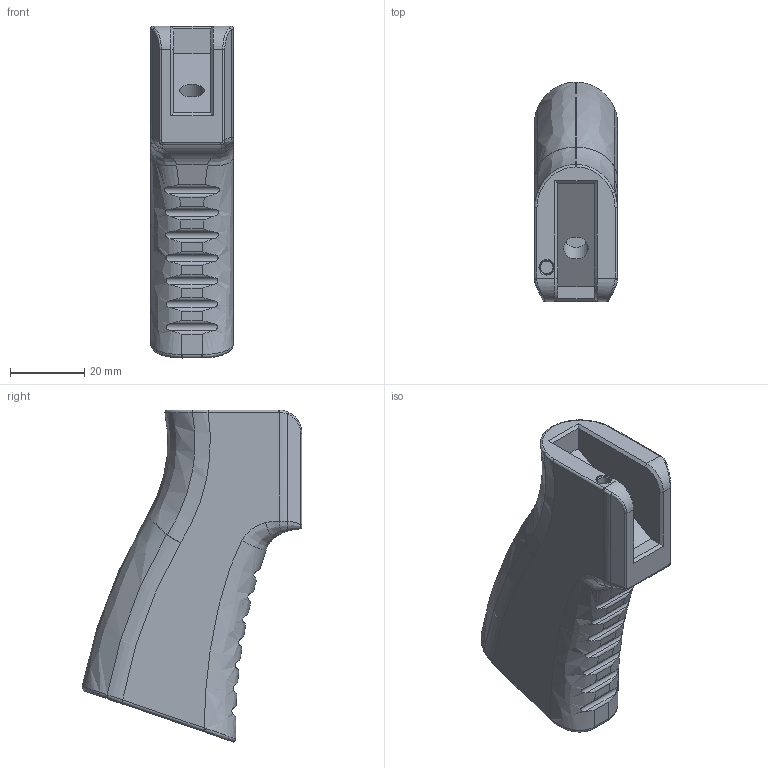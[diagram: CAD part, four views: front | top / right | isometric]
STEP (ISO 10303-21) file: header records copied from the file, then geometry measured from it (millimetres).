
FILE_DESCRIPTION(/* description */ (''),/* implementation_level */ '2;1');
FILE_NAME(/* name */ 'Vulpes Grip.step',/* time_stamp */ '2021-10-04T05:32:21-04:00',/* author */ (''),/* organization */ (''),/* preprocessor_version */ 'ST-DEVELOPER v18.1',/* originating_system */ 'Autodesk Translation Framework v10.10.0.1391',/* authorisation */ '');
FILE_SCHEMA (('AUTOMOTIVE_DESIGN { 1 0 10303 214 3 1 1 }'));
Length unit declared in the file: millimetre
Products named in the file (1): Vulpes Grip
Bounding box: 22.33 x 59.24 x 89.45 mm (x, y, z)
Volume: 33129 mm3; surface area: 16824.8 mm2
Topology: 1 solids, 1 shells, 296 faces, 770 edges, 481 vertices
Faces by surface type: bspline 122, cylinder 79, torus 46, plane 37, sphere 8, cone 4
Full cylindrical faces by diameter (mm): 3.4 x1, 6.8 x1, 14.521 x1, 16.771 x1
Entity records: 14718 total; most frequent: CARTESIAN_POINT 8315, ORIENTED_EDGE 1532, DIRECTION 1026, EDGE_CURVE 766, VERTEX_POINT 481, AXIS2_PLACEMENT_3D 429, B_SPLINE_CURVE_WITH_KNOTS 339, EDGE_LOOP 307
